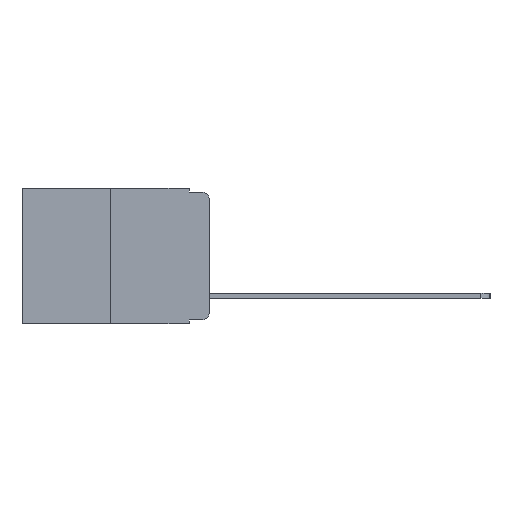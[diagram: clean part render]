
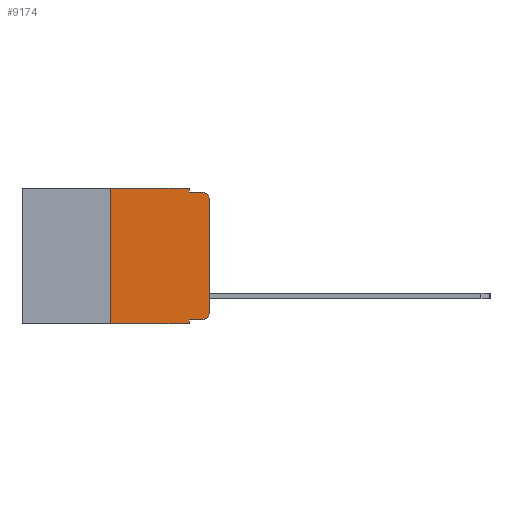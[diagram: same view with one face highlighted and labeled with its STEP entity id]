
A CAD part, left-side view. The second image highlights one B-rep face of the part: STEP entity #9174.
In plain terms, the highlighted planar face has unit normal (-1, 0, 0).
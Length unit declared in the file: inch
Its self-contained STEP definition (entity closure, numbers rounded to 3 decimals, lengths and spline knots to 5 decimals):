
#275 = ORIENTED_EDGE ( 'NONE', *, *, #2612, .T. ) ;
#278 = EDGE_CURVE ( 'NONE', #8805, #11707, #10113, .T. ) ;
#330 = DIRECTION ( 'NONE',  ( 0., 0., -1. ) ) ;
#332 = CARTESIAN_POINT ( 'NONE',  ( 0., 0.473, 0. ) ) ;
#779 = LINE ( 'NONE', #1641, #1705 ) ;
#829 = EDGE_CURVE ( 'NONE', #8162, #8875, #1807, .T. ) ;
#848 = CARTESIAN_POINT ( 'NONE',  ( 0., 0.02, -0.333 ) ) ;
#853 = CARTESIAN_POINT ( 'NONE',  ( 0., 0.051, 0. ) ) ;
#959 = CARTESIAN_POINT ( 'NONE',  ( 0., 0.051, -0.343 ) ) ;
#1155 = VECTOR ( 'NONE', #4229, 39.37008 ) ;
#1215 = ORIENTED_EDGE ( 'NONE', *, *, #12357, .F. ) ;
#1305 = CARTESIAN_POINT ( 'NONE',  ( 0., 0.051, -0.333 ) ) ;
#1641 = CARTESIAN_POINT ( 'NONE',  ( 0., 0.25, 0. ) ) ;
#1705 = VECTOR ( 'NONE', #9415, 39.37008 ) ;
#1755 = LINE ( 'NONE', #7112, #10350 ) ;
#1807 = LINE ( 'NONE', #9153, #12022 ) ;
#2302 = CARTESIAN_POINT ( 'NONE',  ( 0., 0.051, -0.333 ) ) ;
#2594 = DIRECTION ( 'NONE',  ( 1., 0., 0. ) ) ;
#2612 = EDGE_CURVE ( 'NONE', #11550, #9105, #3027, .T. ) ;
#2759 = CARTESIAN_POINT ( 'NONE',  ( 0., 0.25, 0. ) ) ;
#2787 = ORIENTED_EDGE ( 'NONE', *, *, #12337, .T. ) ;
#2887 = VERTEX_POINT ( 'NONE', #2759 ) ;
#3027 = CIRCLE ( 'NONE', #6789, 0.02 ) ;
#3211 = CARTESIAN_POINT ( 'NONE',  ( 0., 0.051, -0.01 ) ) ;
#3465 = LINE ( 'NONE', #332, #1155 ) ;
#3572 = AXIS2_PLACEMENT_3D ( 'NONE', #5027, #11762, #5966 ) ;
#4229 = DIRECTION ( 'NONE',  ( 0., -1., 0. ) ) ;
#4314 = VECTOR ( 'NONE', #11198, 39.37008 ) ;
#4425 = VECTOR ( 'NONE', #8036, 39.37008 ) ;
#4446 = EDGE_CURVE ( 'NONE', #11707, #9105, #11965, .T. ) ;
#4617 = DIRECTION ( 'NONE',  ( 0., 0., -1. ) ) ;
#4700 = ORIENTED_EDGE ( 'NONE', *, *, #6596, .F. ) ;
#4841 = EDGE_CURVE ( 'NONE', #5421, #8011, #6358, .T. ) ;
#4846 = DIRECTION ( 'NONE',  ( 0., -1., 0. ) ) ;
#4941 = CARTESIAN_POINT ( 'NONE',  ( 0., 0., -0.313 ) ) ;
#4980 = EDGE_LOOP ( 'NONE', ( #9980, #275, #10589, #5723, #1215, #8924, #6617, #4700, #2787, #7841 ) ) ;
#5027 = CARTESIAN_POINT ( 'NONE',  ( 0., 0.02, -0.313 ) ) ;
#5306 = CARTESIAN_POINT ( 'NONE',  ( 0., 0.02, -0.03 ) ) ;
#5421 = VERTEX_POINT ( 'NONE', #848 ) ;
#5662 = AXIS2_PLACEMENT_3D ( 'NONE', #8324, #2594, #9317 ) ;
#5723 = ORIENTED_EDGE ( 'NONE', *, *, #278, .F. ) ;
#5831 = EDGE_CURVE ( 'NONE', #8011, #11550, #9859, .T. ) ;
#5840 = VERTEX_POINT ( 'NONE', #1305 ) ;
#5945 = VECTOR ( 'NONE', #6060, 39.37008 ) ;
#5966 = DIRECTION ( 'NONE',  ( 0., 0., -1. ) ) ;
#6060 = DIRECTION ( 'NONE',  ( 0., -1., 0. ) ) ;
#6245 = DIRECTION ( 'NONE',  ( 0., 0., -1. ) ) ;
#6358 = CIRCLE ( 'NONE', #3572, 0.02 ) ;
#6596 = EDGE_CURVE ( 'NONE', #5840, #8875, #1755, .T. ) ;
#6617 = ORIENTED_EDGE ( 'NONE', *, *, #829, .T. ) ;
#6789 = AXIS2_PLACEMENT_3D ( 'NONE', #5306, #12046, #6245 ) ;
#7041 = CARTESIAN_POINT ( 'NONE',  ( 0., 0., 0. ) ) ;
#7112 = CARTESIAN_POINT ( 'NONE',  ( 0., 0.051, 0. ) ) ;
#7219 = FACE_OUTER_BOUND ( 'NONE', #4980, .T. ) ;
#7319 = PLANE ( 'NONE',  #5662 ) ;
#7746 = CARTESIAN_POINT ( 'NONE',  ( 0., 0., -0.03 ) ) ;
#7841 = ORIENTED_EDGE ( 'NONE', *, *, #4841, .T. ) ;
#8011 = VERTEX_POINT ( 'NONE', #4941 ) ;
#8036 = DIRECTION ( 'NONE',  ( 0., 0., 1. ) ) ;
#8162 = VERTEX_POINT ( 'NONE', #10962 ) ;
#8324 = CARTESIAN_POINT ( 'NONE',  ( 0., 0.473, 0. ) ) ;
#8731 = EDGE_CURVE ( 'NONE', #8162, #2887, #779, .T. ) ;
#8805 = VERTEX_POINT ( 'NONE', #9541 ) ;
#8861 = LINE ( 'NONE', #2302, #5945 ) ;
#8875 = VERTEX_POINT ( 'NONE', #959 ) ;
#8924 = ORIENTED_EDGE ( 'NONE', *, *, #8731, .F. ) ;
#9105 = VERTEX_POINT ( 'NONE', #11971 ) ;
#9153 = CARTESIAN_POINT ( 'NONE',  ( 0., 0.473, -0.343 ) ) ;
#9174 = ADVANCED_FACE ( 'NONE', ( #7219 ), #7319, .F. ) ;
#9317 = DIRECTION ( 'NONE',  ( 0., 0., -1. ) ) ;
#9415 = DIRECTION ( 'NONE',  ( 0., 0., 1. ) ) ;
#9516 = VECTOR ( 'NONE', #4617, 39.37008 ) ;
#9541 = CARTESIAN_POINT ( 'NONE',  ( 0., 0.051, 0. ) ) ;
#9859 = LINE ( 'NONE', #7041, #4425 ) ;
#9980 = ORIENTED_EDGE ( 'NONE', *, *, #5831, .T. ) ;
#10113 = LINE ( 'NONE', #853, #9516 ) ;
#10350 = VECTOR ( 'NONE', #330, 39.37008 ) ;
#10589 = ORIENTED_EDGE ( 'NONE', *, *, #4446, .F. ) ;
#10962 = CARTESIAN_POINT ( 'NONE',  ( 0., 0.25, -0.343 ) ) ;
#11198 = DIRECTION ( 'NONE',  ( 0., -1., 0. ) ) ;
#11550 = VERTEX_POINT ( 'NONE', #7746 ) ;
#11707 = VERTEX_POINT ( 'NONE', #3211 ) ;
#11762 = DIRECTION ( 'NONE',  ( -1., 0., 0. ) ) ;
#11965 = LINE ( 'NONE', #12147, #4314 ) ;
#11971 = CARTESIAN_POINT ( 'NONE',  ( 0., 0.02, -0.01 ) ) ;
#12022 = VECTOR ( 'NONE', #4846, 39.37008 ) ;
#12046 = DIRECTION ( 'NONE',  ( -1., 0., 0. ) ) ;
#12147 = CARTESIAN_POINT ( 'NONE',  ( 0., 0.051, -0.01 ) ) ;
#12337 = EDGE_CURVE ( 'NONE', #5840, #5421, #8861, .T. ) ;
#12357 = EDGE_CURVE ( 'NONE', #2887, #8805, #3465, .T. ) ;
